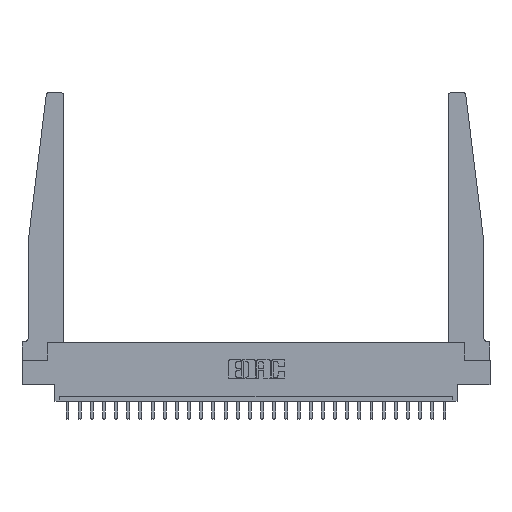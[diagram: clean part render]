
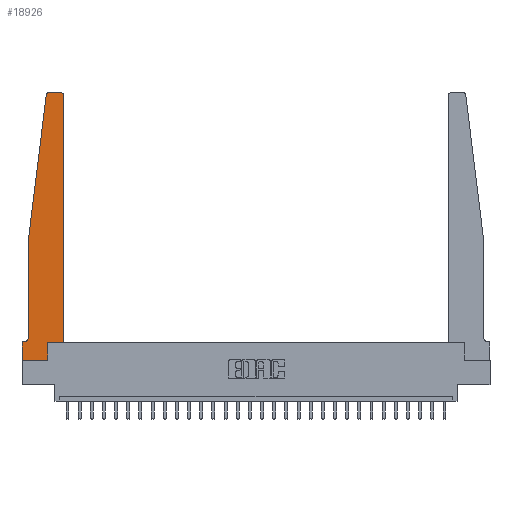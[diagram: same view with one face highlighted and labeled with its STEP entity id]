
A CAD part, top view. The second image highlights one B-rep face of the part: STEP entity #18926.
In plain terms, the highlighted planar face has unit normal (0, 0, 1).
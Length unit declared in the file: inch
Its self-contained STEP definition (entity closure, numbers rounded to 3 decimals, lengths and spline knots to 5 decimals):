
#208 = VECTOR ( 'NONE', #21890, 39.37008 ) ;
#228 = CARTESIAN_POINT ( 'NONE',  ( 0., 0., 0.37 ) ) ;
#269 = DIRECTION ( 'NONE',  ( 0., 1., 0. ) ) ;
#271 = VERTEX_POINT ( 'NONE', #9837 ) ;
#402 = CARTESIAN_POINT ( 'NONE',  ( 0.065, 1.25, 0.37 ) ) ;
#1075 = CARTESIAN_POINT ( 'NONE',  ( 0.425, 2.72, 0.37 ) ) ;
#1222 = CARTESIAN_POINT ( 'NONE',  ( 0., 0.1875, 0.37 ) ) ;
#1316 = CARTESIAN_POINT ( 'NONE',  ( 0.25, 2.75, 0.37 ) ) ;
#1626 = VECTOR ( 'NONE', #2421, 39.37008 ) ;
#1806 = EDGE_CURVE ( 'NONE', #23003, #17731, #7041, .T. ) ;
#2119 = CARTESIAN_POINT ( 'NONE',  ( 0.2605, 0., 0.37 ) ) ;
#2146 = LINE ( 'NONE', #13689, #208 ) ;
#2421 = DIRECTION ( 'NONE',  ( -0.122, -0.992, 0. ) ) ;
#2515 = CARTESIAN_POINT ( 'NONE',  ( 0.24675, 2.72367, 0.37 ) ) ;
#3069 = EDGE_CURVE ( 'NONE', #17953, #271, #8678, .T. ) ;
#3144 = CARTESIAN_POINT ( 'NONE',  ( 0.2605, 0.18, 0.37 ) ) ;
#3171 = VERTEX_POINT ( 'NONE', #1075 ) ;
#3230 = DIRECTION ( 'NONE',  ( -1., 0., 0. ) ) ;
#4192 = CARTESIAN_POINT ( 'NONE',  ( 0.065, 1.25, 0.37 ) ) ;
#4351 = VECTOR ( 'NONE', #17586, 39.37008 ) ;
#4535 = CARTESIAN_POINT ( 'NONE',  ( 0.065, 0.2375, 0.37 ) ) ;
#4664 = DIRECTION ( 'NONE',  ( -1., 0., 0. ) ) ;
#4806 = DIRECTION ( 'NONE',  ( -1., 0., 0. ) ) ;
#5164 = AXIS2_PLACEMENT_3D ( 'NONE', #12652, #11533, #22887 ) ;
#5363 = CARTESIAN_POINT ( 'NONE',  ( 0.27653, 2.75, 0.37 ) ) ;
#5436 = DIRECTION ( 'NONE',  ( 1., 0., 0. ) ) ;
#5698 = FACE_OUTER_BOUND ( 'NONE', #13107, .T. ) ;
#6767 = ORIENTED_EDGE ( 'NONE', *, *, #1806, .T. ) ;
#6784 = CARTESIAN_POINT ( 'NONE',  ( 0.425, 0.18, 0.37 ) ) ;
#7041 = CIRCLE ( 'NONE', #26388, 0.03 ) ;
#8097 = CARTESIAN_POINT ( 'NONE',  ( 0., 0.1875, 0.37 ) ) ;
#8190 = AXIS2_PLACEMENT_3D ( 'NONE', #1222, #9752, #5436 ) ;
#8439 = ORIENTED_EDGE ( 'NONE', *, *, #3069, .T. ) ;
#8678 = LINE ( 'NONE', #6784, #22549 ) ;
#8954 = ORIENTED_EDGE ( 'NONE', *, *, #11593, .T. ) ;
#8970 = EDGE_CURVE ( 'NONE', #9082, #10523, #9102, .T. ) ;
#9082 = VERTEX_POINT ( 'NONE', #4535 ) ;
#9102 = CIRCLE ( 'NONE', #22849, 0.05 ) ;
#9156 = EDGE_CURVE ( 'NONE', #16501, #9082, #19329, .T. ) ;
#9578 = VECTOR ( 'NONE', #269, 39.37008 ) ;
#9752 = DIRECTION ( 'NONE',  ( 0., 0., 1. ) ) ;
#9837 = CARTESIAN_POINT ( 'NONE',  ( 0.425, 0.18, 0.37 ) ) ;
#10114 = ORIENTED_EDGE ( 'NONE', *, *, #18197, .T. ) ;
#10523 = VERTEX_POINT ( 'NONE', #11584 ) ;
#11533 = DIRECTION ( 'NONE',  ( 0., 0., 1. ) ) ;
#11556 = CARTESIAN_POINT ( 'NONE',  ( 0.2605, 0.18, 0.37 ) ) ;
#11584 = CARTESIAN_POINT ( 'NONE',  ( 0.015, 0.1875, 0.37 ) ) ;
#11592 = VECTOR ( 'NONE', #4664, 39.37008 ) ;
#11593 = EDGE_CURVE ( 'NONE', #11885, #14845, #2146, .T. ) ;
#11800 = EDGE_CURVE ( 'NONE', #20897, #23003, #13618, .T. ) ;
#11885 = VERTEX_POINT ( 'NONE', #8097 ) ;
#12154 = VERTEX_POINT ( 'NONE', #2119 ) ;
#12652 = CARTESIAN_POINT ( 'NONE',  ( 0.395, 2.72, 0.37 ) ) ;
#12700 = ORIENTED_EDGE ( 'NONE', *, *, #22757, .T. ) ;
#13107 = EDGE_LOOP ( 'NONE', ( #13470, #6767, #17134, #22246, #23934, #10114, #8954, #12700, #13403, #8439, #19860, #23505 ) ) ;
#13403 = ORIENTED_EDGE ( 'NONE', *, *, #21656, .T. ) ;
#13470 = ORIENTED_EDGE ( 'NONE', *, *, #11800, .T. ) ;
#13618 = LINE ( 'NONE', #1316, #22182 ) ;
#13689 = CARTESIAN_POINT ( 'NONE',  ( 0., 0., 0.37 ) ) ;
#14845 = VERTEX_POINT ( 'NONE', #22537 ) ;
#14899 = DIRECTION ( 'NONE',  ( 0., 0., -1. ) ) ;
#14989 = DIRECTION ( 'NONE',  ( 1., 0., 0. ) ) ;
#15678 = PLANE ( 'NONE',  #8190 ) ;
#16063 = CARTESIAN_POINT ( 'NONE',  ( 0.425, 0.18, 0.37 ) ) ;
#16285 = LINE ( 'NONE', #228, #26604 ) ;
#16438 = EDGE_CURVE ( 'NONE', #271, #3171, #22508, .T. ) ;
#16501 = VERTEX_POINT ( 'NONE', #4192 ) ;
#16579 = CARTESIAN_POINT ( 'NONE',  ( 0.395, 2.75, 0.37 ) ) ;
#16634 = CARTESIAN_POINT ( 'NONE',  ( 0.015, 0.2375, 0.37 ) ) ;
#16841 = CARTESIAN_POINT ( 'NONE',  ( 0.27653, 2.72, 0.37 ) ) ;
#17134 = ORIENTED_EDGE ( 'NONE', *, *, #20441, .T. ) ;
#17586 = DIRECTION ( 'NONE',  ( 0., -1., 0. ) ) ;
#17731 = VERTEX_POINT ( 'NONE', #2515 ) ;
#17953 = VERTEX_POINT ( 'NONE', #11556 ) ;
#18024 = CIRCLE ( 'NONE', #5164, 0.03 ) ;
#18197 = EDGE_CURVE ( 'NONE', #10523, #11885, #18673, .T. ) ;
#18673 = LINE ( 'NONE', #20406, #11592 ) ;
#18926 = ADVANCED_FACE ( 'NONE', ( #5698 ), #15678, .T. ) ;
#19329 = LINE ( 'NONE', #21367, #4351 ) ;
#19619 = EDGE_CURVE ( 'NONE', #3171, #20897, #18024, .T. ) ;
#19860 = ORIENTED_EDGE ( 'NONE', *, *, #16438, .T. ) ;
#20406 = CARTESIAN_POINT ( 'NONE',  ( 0.065, 0.1875, 0.37 ) ) ;
#20441 = EDGE_CURVE ( 'NONE', #17731, #16501, #22653, .T. ) ;
#20897 = VERTEX_POINT ( 'NONE', #16579 ) ;
#21367 = CARTESIAN_POINT ( 'NONE',  ( 0.065, 1.25, 0.37 ) ) ;
#21607 = LINE ( 'NONE', #3144, #23567 ) ;
#21656 = EDGE_CURVE ( 'NONE', #12154, #17953, #21607, .T. ) ;
#21890 = DIRECTION ( 'NONE',  ( 0., -1., 0. ) ) ;
#22182 = VECTOR ( 'NONE', #3230, 39.37008 ) ;
#22246 = ORIENTED_EDGE ( 'NONE', *, *, #9156, .T. ) ;
#22508 = LINE ( 'NONE', #16063, #9578 ) ;
#22537 = CARTESIAN_POINT ( 'NONE',  ( 0., 0., 0.37 ) ) ;
#22549 = VECTOR ( 'NONE', #14989, 39.37008 ) ;
#22653 = LINE ( 'NONE', #402, #1626 ) ;
#22757 = EDGE_CURVE ( 'NONE', #14845, #12154, #16285, .T. ) ;
#22849 = AXIS2_PLACEMENT_3D ( 'NONE', #16634, #14899, #4806 ) ;
#22887 = DIRECTION ( 'NONE',  ( 1., 0., 0. ) ) ;
#23003 = VERTEX_POINT ( 'NONE', #5363 ) ;
#23036 = DIRECTION ( 'NONE',  ( 1., 0., 0. ) ) ;
#23505 = ORIENTED_EDGE ( 'NONE', *, *, #19619, .T. ) ;
#23567 = VECTOR ( 'NONE', #23913, 39.37008 ) ;
#23913 = DIRECTION ( 'NONE',  ( 0., 1., 0. ) ) ;
#23934 = ORIENTED_EDGE ( 'NONE', *, *, #8970, .T. ) ;
#24931 = DIRECTION ( 'NONE',  ( 0., 0., 1. ) ) ;
#25030 = DIRECTION ( 'NONE',  ( 1., 0., 0. ) ) ;
#26388 = AXIS2_PLACEMENT_3D ( 'NONE', #16841, #24931, #23036 ) ;
#26604 = VECTOR ( 'NONE', #25030, 39.37008 ) ;
